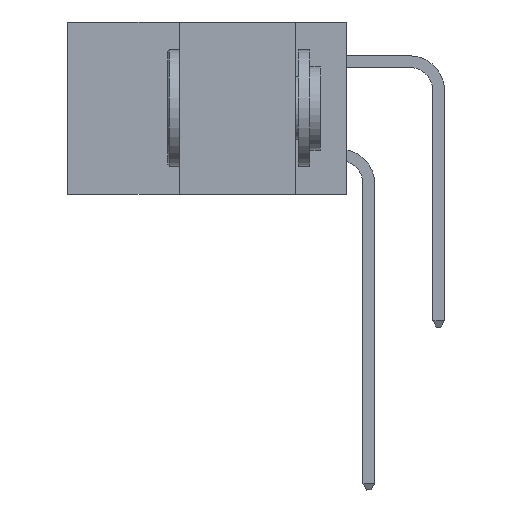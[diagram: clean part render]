
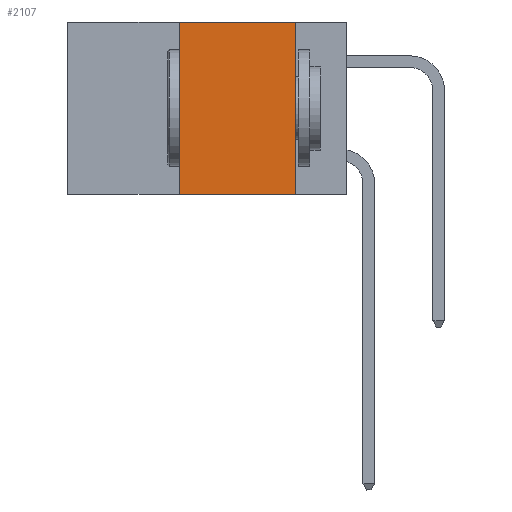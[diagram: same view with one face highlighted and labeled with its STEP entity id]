
A CAD part, left-side view. The second image highlights one B-rep face of the part: STEP entity #2107.
In plain terms, the highlighted planar face has unit normal (-1, 0, 0).
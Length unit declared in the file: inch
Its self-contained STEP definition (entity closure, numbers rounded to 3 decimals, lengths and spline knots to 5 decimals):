
#134 = VECTOR ( 'NONE', #3993, 39.37008 ) ;
#201 = DIRECTION ( 'NONE',  ( 0., 0., 1. ) ) ;
#2107 = ADVANCED_FACE ( 'NONE', ( #15626 ), #17617, .F. ) ;
#2707 = VERTEX_POINT ( 'NONE', #9256 ) ;
#3183 = VERTEX_POINT ( 'NONE', #19828 ) ;
#3335 = CARTESIAN_POINT ( 'NONE',  ( 0., 0.11, 0. ) ) ;
#3993 = DIRECTION ( 'NONE',  ( 0., -1., 0. ) ) ;
#4117 = DIRECTION ( 'NONE',  ( 0., -1., 0. ) ) ;
#4153 = ORIENTED_EDGE ( 'NONE', *, *, #21569, .F. ) ;
#4592 = VECTOR ( 'NONE', #4117, 39.37008 ) ;
#4788 = EDGE_CURVE ( 'NONE', #2707, #10000, #8853, .T. ) ;
#5627 = DIRECTION ( 'NONE',  ( 1., 0., 0. ) ) ;
#6879 = ORIENTED_EDGE ( 'NONE', *, *, #22069, .F. ) ;
#7103 = LINE ( 'NONE', #21791, #134 ) ;
#7145 = LINE ( 'NONE', #3335, #20782 ) ;
#7197 = DIRECTION ( 'NONE',  ( 0., 0., -1. ) ) ;
#8030 = EDGE_LOOP ( 'NONE', ( #6879, #19593, #4153, #8779 ) ) ;
#8779 = ORIENTED_EDGE ( 'NONE', *, *, #22906, .T. ) ;
#8853 = LINE ( 'NONE', #18813, #4592 ) ;
#8885 = AXIS2_PLACEMENT_3D ( 'NONE', #21768, #5627, #7197 ) ;
#9256 = CARTESIAN_POINT ( 'NONE',  ( 0., 0.36, 0. ) ) ;
#10000 = VERTEX_POINT ( 'NONE', #21016 ) ;
#12132 = LINE ( 'NONE', #18001, #19670 ) ;
#12576 = VERTEX_POINT ( 'NONE', #15719 ) ;
#15626 = FACE_OUTER_BOUND ( 'NONE', #8030, .T. ) ;
#15719 = CARTESIAN_POINT ( 'NONE',  ( 0., 0.36, -0.37 ) ) ;
#15780 = DIRECTION ( 'NONE',  ( 0., 0., -1. ) ) ;
#17617 = PLANE ( 'NONE',  #8885 ) ;
#18001 = CARTESIAN_POINT ( 'NONE',  ( 0., 0.36, 0. ) ) ;
#18813 = CARTESIAN_POINT ( 'NONE',  ( 0., 0.6, 0. ) ) ;
#19593 = ORIENTED_EDGE ( 'NONE', *, *, #4788, .F. ) ;
#19670 = VECTOR ( 'NONE', #201, 39.37008 ) ;
#19828 = CARTESIAN_POINT ( 'NONE',  ( 0., 0.11, -0.37 ) ) ;
#20782 = VECTOR ( 'NONE', #15780, 39.37008 ) ;
#21016 = CARTESIAN_POINT ( 'NONE',  ( 0., 0.11, 0. ) ) ;
#21569 = EDGE_CURVE ( 'NONE', #12576, #2707, #12132, .T. ) ;
#21768 = CARTESIAN_POINT ( 'NONE',  ( 0., 0.6, 0. ) ) ;
#21791 = CARTESIAN_POINT ( 'NONE',  ( 0., 0.6, -0.37 ) ) ;
#22069 = EDGE_CURVE ( 'NONE', #10000, #3183, #7145, .T. ) ;
#22906 = EDGE_CURVE ( 'NONE', #12576, #3183, #7103, .T. ) ;
